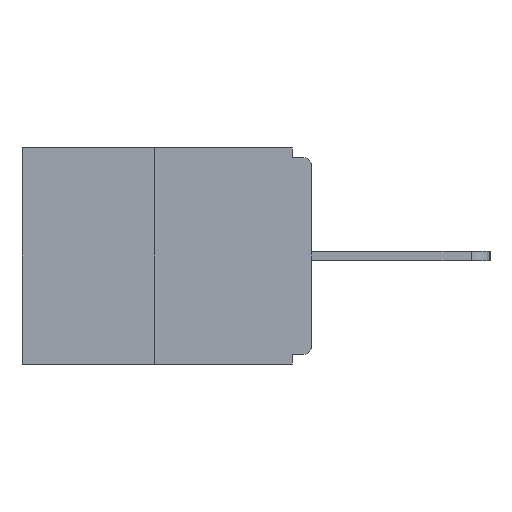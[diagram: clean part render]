
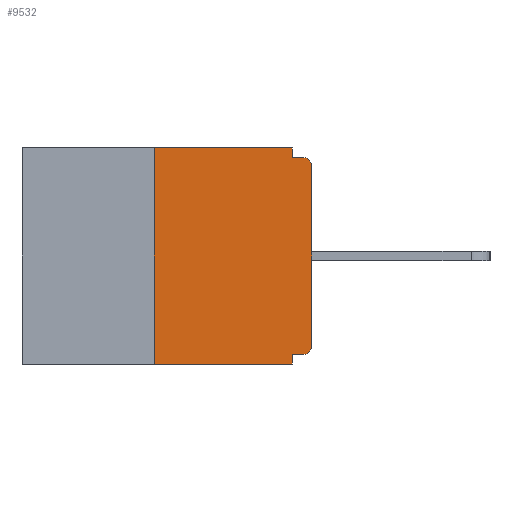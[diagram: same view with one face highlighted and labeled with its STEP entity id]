
A CAD part, left-side view. The second image highlights one B-rep face of the part: STEP entity #9532.
In plain terms, the highlighted planar face has unit normal (-1, 0, 0).
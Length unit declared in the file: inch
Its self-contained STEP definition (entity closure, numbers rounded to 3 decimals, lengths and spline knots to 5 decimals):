
#144 = LINE ( 'NONE', #5226, #3714 ) ;
#412 = VERTEX_POINT ( 'NONE', #1001 ) ;
#528 = LINE ( 'NONE', #11935, #10652 ) ;
#557 = VERTEX_POINT ( 'NONE', #15907 ) ;
#564 = DIRECTION ( 'NONE',  ( 1., 0., 0. ) ) ;
#811 = CARTESIAN_POINT ( 'NONE',  ( 0., 0.46, 0. ) ) ;
#1001 = CARTESIAN_POINT ( 'NONE',  ( 0., 0., -0.03 ) ) ;
#1186 = CARTESIAN_POINT ( 'NONE',  ( 0., 0.015, -0.328 ) ) ;
#1361 = EDGE_CURVE ( 'NONE', #13213, #6407, #15440, .T. ) ;
#1372 = ORIENTED_EDGE ( 'NONE', *, *, #5356, .T. ) ;
#1564 = EDGE_CURVE ( 'NONE', #557, #412, #10003, .T. ) ;
#1903 = CARTESIAN_POINT ( 'NONE',  ( 0., 0.015, -0.03 ) ) ;
#2211 = ORIENTED_EDGE ( 'NONE', *, *, #1361, .F. ) ;
#2263 = CARTESIAN_POINT ( 'NONE',  ( 0., 0., 0. ) ) ;
#2305 = CARTESIAN_POINT ( 'NONE',  ( 0., 0.031, -0.343 ) ) ;
#2318 = CARTESIAN_POINT ( 'NONE',  ( 0., 0.015, -0.015 ) ) ;
#2390 = DIRECTION ( 'NONE',  ( 0., 0., -1. ) ) ;
#2451 = DIRECTION ( 'NONE',  ( -1., 0., 0. ) ) ;
#2599 = DIRECTION ( 'NONE',  ( 0., -1., 0. ) ) ;
#2656 = EDGE_CURVE ( 'NONE', #5571, #557, #5065, .T. ) ;
#3158 = ORIENTED_EDGE ( 'NONE', *, *, #14029, .F. ) ;
#3684 = CARTESIAN_POINT ( 'NONE',  ( 0., 0.25, 0. ) ) ;
#3714 = VECTOR ( 'NONE', #11630, 39.37008 ) ;
#4045 = EDGE_LOOP ( 'NONE', ( #3158, #11374, #1372, #15757, #5210, #15884, #6943, #4729, #8625, #2211 ) ) ;
#4327 = VERTEX_POINT ( 'NONE', #3684 ) ;
#4729 = ORIENTED_EDGE ( 'NONE', *, *, #12308, .T. ) ;
#5065 = CIRCLE ( 'NONE', #7714, 0.015 ) ;
#5210 = ORIENTED_EDGE ( 'NONE', *, *, #13968, .F. ) ;
#5226 = CARTESIAN_POINT ( 'NONE',  ( 0., 0., -0.328 ) ) ;
#5356 = EDGE_CURVE ( 'NONE', #6419, #7599, #528, .T. ) ;
#5571 = VERTEX_POINT ( 'NONE', #1186 ) ;
#5797 = DIRECTION ( 'NONE',  ( 0., -1., 0. ) ) ;
#6201 = CARTESIAN_POINT ( 'NONE',  ( 0., 0.031, -0.328 ) ) ;
#6381 = LINE ( 'NONE', #2305, #15349 ) ;
#6407 = VERTEX_POINT ( 'NONE', #13081 ) ;
#6419 = VERTEX_POINT ( 'NONE', #6661 ) ;
#6598 = CARTESIAN_POINT ( 'NONE',  ( 0., 0.031, 0. ) ) ;
#6622 = CIRCLE ( 'NONE', #15938, 0.015 ) ;
#6661 = CARTESIAN_POINT ( 'NONE',  ( 0., 0.25, -0.343 ) ) ;
#6703 = VERTEX_POINT ( 'NONE', #2318 ) ;
#6809 = AXIS2_PLACEMENT_3D ( 'NONE', #811, #564, #10715 ) ;
#6943 = ORIENTED_EDGE ( 'NONE', *, *, #1564, .T. ) ;
#7338 = CARTESIAN_POINT ( 'NONE',  ( 0., 0., -0.015 ) ) ;
#7503 = LINE ( 'NONE', #7338, #7632 ) ;
#7599 = VERTEX_POINT ( 'NONE', #15667 ) ;
#7632 = VECTOR ( 'NONE', #2599, 39.37008 ) ;
#7692 = CARTESIAN_POINT ( 'NONE',  ( 0., 0.015, -0.313 ) ) ;
#7714 = AXIS2_PLACEMENT_3D ( 'NONE', #7692, #2451, #9942 ) ;
#8625 = ORIENTED_EDGE ( 'NONE', *, *, #10350, .F. ) ;
#9266 = DIRECTION ( 'NONE',  ( 0., 0., -1. ) ) ;
#9532 = ADVANCED_FACE ( 'NONE', ( #13641 ), #15890, .F. ) ;
#9556 = EDGE_CURVE ( 'NONE', #6419, #4327, #10217, .T. ) ;
#9560 = EDGE_CURVE ( 'NONE', #11250, #7599, #6381, .T. ) ;
#9942 = DIRECTION ( 'NONE',  ( 0., 0., -1. ) ) ;
#10003 = LINE ( 'NONE', #2263, #14864 ) ;
#10048 = CARTESIAN_POINT ( 'NONE',  ( 0., 0.25, 0. ) ) ;
#10095 = VECTOR ( 'NONE', #5797, 39.37008 ) ;
#10217 = LINE ( 'NONE', #10048, #12135 ) ;
#10350 = EDGE_CURVE ( 'NONE', #6407, #6703, #7503, .T. ) ;
#10652 = VECTOR ( 'NONE', #15777, 39.37008 ) ;
#10715 = DIRECTION ( 'NONE',  ( 0., 0., -1. ) ) ;
#11250 = VERTEX_POINT ( 'NONE', #6201 ) ;
#11374 = ORIENTED_EDGE ( 'NONE', *, *, #9556, .F. ) ;
#11630 = DIRECTION ( 'NONE',  ( 0., 1., 0. ) ) ;
#11935 = CARTESIAN_POINT ( 'NONE',  ( 0., 0.46, -0.343 ) ) ;
#12042 = LINE ( 'NONE', #14632, #10095 ) ;
#12055 = DIRECTION ( 'NONE',  ( -1., 0., 0. ) ) ;
#12135 = VECTOR ( 'NONE', #13889, 39.37008 ) ;
#12137 = DIRECTION ( 'NONE',  ( 0., 0., -1. ) ) ;
#12308 = EDGE_CURVE ( 'NONE', #412, #6703, #6622, .T. ) ;
#12323 = CARTESIAN_POINT ( 'NONE',  ( 0., 0.031, 0. ) ) ;
#12998 = VECTOR ( 'NONE', #9266, 39.37008 ) ;
#13081 = CARTESIAN_POINT ( 'NONE',  ( 0., 0.031, -0.015 ) ) ;
#13213 = VERTEX_POINT ( 'NONE', #12323 ) ;
#13641 = FACE_OUTER_BOUND ( 'NONE', #4045, .T. ) ;
#13889 = DIRECTION ( 'NONE',  ( 0., 0., 1. ) ) ;
#13968 = EDGE_CURVE ( 'NONE', #5571, #11250, #144, .T. ) ;
#14029 = EDGE_CURVE ( 'NONE', #4327, #13213, #12042, .T. ) ;
#14632 = CARTESIAN_POINT ( 'NONE',  ( 0., 0.46, 0. ) ) ;
#14864 = VECTOR ( 'NONE', #15264, 39.37008 ) ;
#15264 = DIRECTION ( 'NONE',  ( 0., 0., 1. ) ) ;
#15349 = VECTOR ( 'NONE', #2390, 39.37008 ) ;
#15440 = LINE ( 'NONE', #6598, #12998 ) ;
#15667 = CARTESIAN_POINT ( 'NONE',  ( 0., 0.031, -0.343 ) ) ;
#15757 = ORIENTED_EDGE ( 'NONE', *, *, #9560, .F. ) ;
#15777 = DIRECTION ( 'NONE',  ( 0., -1., 0. ) ) ;
#15884 = ORIENTED_EDGE ( 'NONE', *, *, #2656, .T. ) ;
#15890 = PLANE ( 'NONE',  #6809 ) ;
#15907 = CARTESIAN_POINT ( 'NONE',  ( 0., 0., -0.313 ) ) ;
#15938 = AXIS2_PLACEMENT_3D ( 'NONE', #1903, #12055, #12137 ) ;
